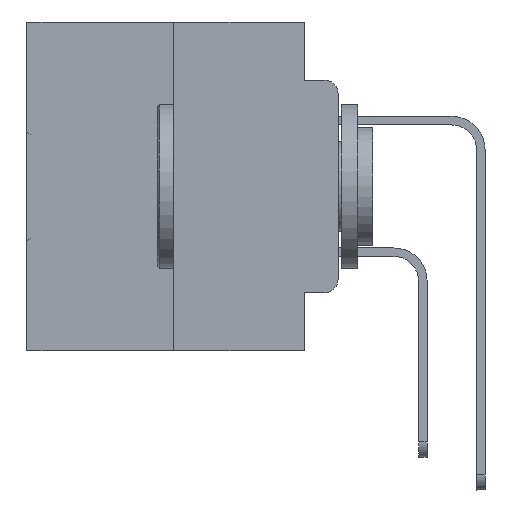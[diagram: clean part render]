
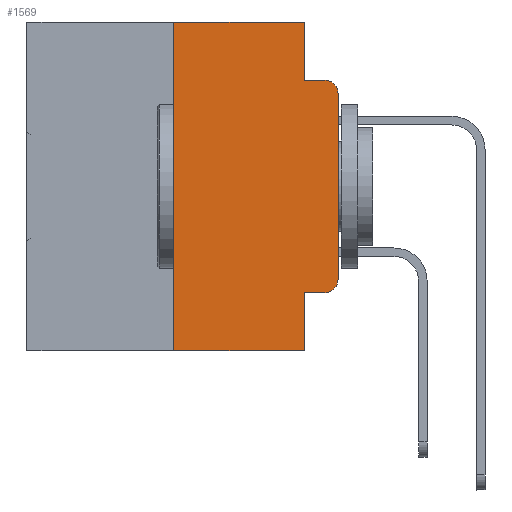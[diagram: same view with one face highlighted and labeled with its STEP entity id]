
A CAD part, left-side view. The second image highlights one B-rep face of the part: STEP entity #1569.
In plain terms, the highlighted planar face has unit normal (-1, 0, 0).
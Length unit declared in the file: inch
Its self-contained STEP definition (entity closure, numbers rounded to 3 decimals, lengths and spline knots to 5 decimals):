
#17 = ORIENTED_EDGE ( 'NONE', *, *, #12670, .F. ) ;
#133 = DIRECTION ( 'NONE',  ( 0., -1., 0. ) ) ;
#239 = DIRECTION ( 'NONE',  ( 0., 0., -1. ) ) ;
#374 = CARTESIAN_POINT ( 'NONE',  ( 0., 0.02, -0.1085 ) ) ;
#711 = CARTESIAN_POINT ( 'NONE',  ( 0., 0.02, -0.3915 ) ) ;
#1569 = ADVANCED_FACE ( 'NONE', ( #22019 ), #14230, .F. ) ;
#1685 = VECTOR ( 'NONE', #239, 39.37008 ) ;
#1735 = DIRECTION ( 'NONE',  ( 0., 0., -1. ) ) ;
#2175 = CARTESIAN_POINT ( 'NONE',  ( 0., 0.25, -0.5 ) ) ;
#2364 = DIRECTION ( 'NONE',  ( 0., 0., 1. ) ) ;
#2410 = DIRECTION ( 'NONE',  ( 0., -1., 0. ) ) ;
#2762 = EDGE_CURVE ( 'NONE', #32863, #14907, #20737, .T. ) ;
#2868 = CARTESIAN_POINT ( 'NONE',  ( 0., 0.473, 0. ) ) ;
#2933 = ORIENTED_EDGE ( 'NONE', *, *, #13713, .T. ) ;
#3045 = DIRECTION ( 'NONE',  ( 0., 0., -1. ) ) ;
#3132 = LINE ( 'NONE', #20595, #16198 ) ;
#3178 = VECTOR ( 'NONE', #26474, 39.37008 ) ;
#3184 = EDGE_CURVE ( 'NONE', #14315, #14907, #23134, .T. ) ;
#3363 = DIRECTION ( 'NONE',  ( 0., 0., -1. ) ) ;
#4549 = ORIENTED_EDGE ( 'NONE', *, *, #21329, .T. ) ;
#4619 = DIRECTION ( 'NONE',  ( 1., 0., 0. ) ) ;
#6147 = CIRCLE ( 'NONE', #24573, 0.02 ) ;
#6308 = VERTEX_POINT ( 'NONE', #15398 ) ;
#6478 = LINE ( 'NONE', #15720, #26458 ) ;
#8216 = VERTEX_POINT ( 'NONE', #32642 ) ;
#8670 = ORIENTED_EDGE ( 'NONE', *, *, #2762, .F. ) ;
#8969 = CARTESIAN_POINT ( 'NONE',  ( 0., 0.051, 0. ) ) ;
#9320 = CARTESIAN_POINT ( 'NONE',  ( 0., 0.02, -0.0885 ) ) ;
#10264 = DIRECTION ( 'NONE',  ( 0., 0., -1. ) ) ;
#12454 = CARTESIAN_POINT ( 'NONE',  ( 0., 0.051, -0.4115 ) ) ;
#12670 = EDGE_CURVE ( 'NONE', #21545, #29922, #27316, .T. ) ;
#13162 = ORIENTED_EDGE ( 'NONE', *, *, #18490, .F. ) ;
#13389 = VERTEX_POINT ( 'NONE', #16301 ) ;
#13713 = EDGE_CURVE ( 'NONE', #30768, #13389, #16292, .T. ) ;
#13971 = ORIENTED_EDGE ( 'NONE', *, *, #15026, .F. ) ;
#14230 = PLANE ( 'NONE',  #22189 ) ;
#14315 = VERTEX_POINT ( 'NONE', #2175 ) ;
#14368 = EDGE_CURVE ( 'NONE', #6308, #23155, #22721, .T. ) ;
#14907 = VERTEX_POINT ( 'NONE', #17555 ) ;
#15026 = EDGE_CURVE ( 'NONE', #14315, #21545, #3132, .T. ) ;
#15398 = CARTESIAN_POINT ( 'NONE',  ( 0., 0.051, -0.0885 ) ) ;
#15486 = VECTOR ( 'NONE', #33043, 39.37008 ) ;
#15720 = CARTESIAN_POINT ( 'NONE',  ( 0., 0.051, -0.4115 ) ) ;
#15843 = VECTOR ( 'NONE', #2410, 39.37008 ) ;
#16198 = VECTOR ( 'NONE', #2364, 39.37008 ) ;
#16292 = LINE ( 'NONE', #30334, #15486 ) ;
#16301 = CARTESIAN_POINT ( 'NONE',  ( 0., 0., -0.1085 ) ) ;
#17203 = AXIS2_PLACEMENT_3D ( 'NONE', #374, #18653, #3045 ) ;
#17555 = CARTESIAN_POINT ( 'NONE',  ( 0., 0.051, -0.5 ) ) ;
#18036 = CARTESIAN_POINT ( 'NONE',  ( 0., 0.051, -0.0885 ) ) ;
#18168 = EDGE_LOOP ( 'NONE', ( #2933, #4549, #18428, #13162, #17, #13971, #28595, #8670, #29407, #30865 ) ) ;
#18428 = ORIENTED_EDGE ( 'NONE', *, *, #14368, .F. ) ;
#18490 = EDGE_CURVE ( 'NONE', #29922, #6308, #29392, .T. ) ;
#18653 = DIRECTION ( 'NONE',  ( -1., 0., 0. ) ) ;
#18971 = DIRECTION ( 'NONE',  ( -1., 0., 0. ) ) ;
#20595 = CARTESIAN_POINT ( 'NONE',  ( 0., 0.25, 0. ) ) ;
#20737 = LINE ( 'NONE', #8969, #33705 ) ;
#21329 = EDGE_CURVE ( 'NONE', #13389, #23155, #27567, .T. ) ;
#21545 = VERTEX_POINT ( 'NONE', #27264 ) ;
#22019 = FACE_OUTER_BOUND ( 'NONE', #18168, .T. ) ;
#22189 = AXIS2_PLACEMENT_3D ( 'NONE', #2868, #4619, #1735 ) ;
#22721 = LINE ( 'NONE', #18036, #15843 ) ;
#23134 = LINE ( 'NONE', #27358, #3178 ) ;
#23155 = VERTEX_POINT ( 'NONE', #9320 ) ;
#23303 = CARTESIAN_POINT ( 'NONE',  ( 0., 0.051, 0. ) ) ;
#23625 = CARTESIAN_POINT ( 'NONE',  ( 0., 0.051, 0. ) ) ;
#24573 = AXIS2_PLACEMENT_3D ( 'NONE', #711, #18971, #3363 ) ;
#26454 = CARTESIAN_POINT ( 'NONE',  ( 0., 0.473, 0. ) ) ;
#26458 = VECTOR ( 'NONE', #133, 39.37008 ) ;
#26474 = DIRECTION ( 'NONE',  ( 0., -1., 0. ) ) ;
#27264 = CARTESIAN_POINT ( 'NONE',  ( 0., 0.25, 0. ) ) ;
#27316 = LINE ( 'NONE', #26454, #32605 ) ;
#27358 = CARTESIAN_POINT ( 'NONE',  ( 0., 0.473, -0.5 ) ) ;
#27567 = CIRCLE ( 'NONE', #17203, 0.02 ) ;
#28595 = ORIENTED_EDGE ( 'NONE', *, *, #3184, .T. ) ;
#29042 = DIRECTION ( 'NONE',  ( 0., -1., 0. ) ) ;
#29392 = LINE ( 'NONE', #23625, #1685 ) ;
#29407 = ORIENTED_EDGE ( 'NONE', *, *, #33069, .T. ) ;
#29922 = VERTEX_POINT ( 'NONE', #23303 ) ;
#30334 = CARTESIAN_POINT ( 'NONE',  ( 0., 0., 0. ) ) ;
#30768 = VERTEX_POINT ( 'NONE', #31887 ) ;
#30865 = ORIENTED_EDGE ( 'NONE', *, *, #31316, .T. ) ;
#31316 = EDGE_CURVE ( 'NONE', #8216, #30768, #6147, .T. ) ;
#31887 = CARTESIAN_POINT ( 'NONE',  ( 0., 0., -0.3915 ) ) ;
#32605 = VECTOR ( 'NONE', #29042, 39.37008 ) ;
#32642 = CARTESIAN_POINT ( 'NONE',  ( 0., 0.02, -0.4115 ) ) ;
#32863 = VERTEX_POINT ( 'NONE', #12454 ) ;
#33043 = DIRECTION ( 'NONE',  ( 0., 0., 1. ) ) ;
#33069 = EDGE_CURVE ( 'NONE', #32863, #8216, #6478, .T. ) ;
#33705 = VECTOR ( 'NONE', #10264, 39.37008 ) ;
